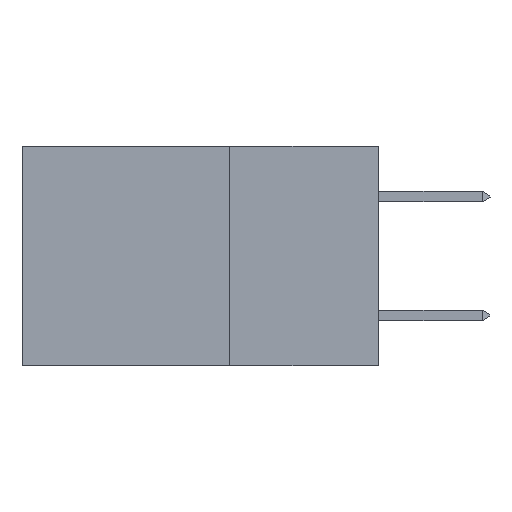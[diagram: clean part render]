
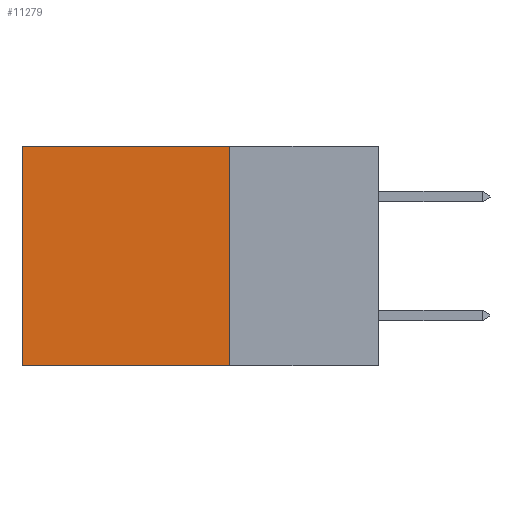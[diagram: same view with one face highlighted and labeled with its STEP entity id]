
A CAD part, left-side view. The second image highlights one B-rep face of the part: STEP entity #11279.
In plain terms, the highlighted planar face has unit normal (-1, 0, 0).
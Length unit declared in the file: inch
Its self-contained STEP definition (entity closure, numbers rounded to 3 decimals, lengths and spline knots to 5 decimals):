
#755 = VERTEX_POINT ( 'NONE', #5905 ) ;
#1146 = DIRECTION ( 'NONE',  ( 0., 0., -1. ) ) ;
#1419 = AXIS2_PLACEMENT_3D ( 'NONE', #7043, #1528, #3377 ) ;
#1528 = DIRECTION ( 'NONE',  ( 1., 0., 0. ) ) ;
#1581 = VECTOR ( 'NONE', #1146, 39.37008 ) ;
#1750 = VECTOR ( 'NONE', #7719, 39.37008 ) ;
#2320 = VECTOR ( 'NONE', #4687, 39.37008 ) ;
#2841 = FACE_OUTER_BOUND ( 'NONE', #6956, .T. ) ;
#2932 = VERTEX_POINT ( 'NONE', #9448 ) ;
#3377 = DIRECTION ( 'NONE',  ( 0., 0., -1. ) ) ;
#3832 = ORIENTED_EDGE ( 'NONE', *, *, #9531, .T. ) ;
#4019 = VERTEX_POINT ( 'NONE', #7221 ) ;
#4687 = DIRECTION ( 'NONE',  ( 0., 1., 0. ) ) ;
#5283 = ORIENTED_EDGE ( 'NONE', *, *, #6499, .F. ) ;
#5541 = ORIENTED_EDGE ( 'NONE', *, *, #7902, .T. ) ;
#5762 = CARTESIAN_POINT ( 'NONE',  ( 0.298, 0.6, 0. ) ) ;
#5766 = CARTESIAN_POINT ( 'NONE',  ( 0.298, 0.25, -0.37 ) ) ;
#5805 = CARTESIAN_POINT ( 'NONE',  ( 0.298, 0.6, -0.37 ) ) ;
#5905 = CARTESIAN_POINT ( 'NONE',  ( 0.298, 0.6, 0. ) ) ;
#6098 = CARTESIAN_POINT ( 'NONE',  ( 0.298, 0.25, 0. ) ) ;
#6193 = PLANE ( 'NONE',  #1419 ) ;
#6499 = EDGE_CURVE ( 'NONE', #2932, #9592, #7952, .T. ) ;
#6956 = EDGE_LOOP ( 'NONE', ( #3832, #5283, #9383, #5541 ) ) ;
#7043 = CARTESIAN_POINT ( 'NONE',  ( 0.298, 0.25, 0. ) ) ;
#7221 = CARTESIAN_POINT ( 'NONE',  ( 0.298, 0.25, 0. ) ) ;
#7719 = DIRECTION ( 'NONE',  ( 0., 1., 0. ) ) ;
#7902 = EDGE_CURVE ( 'NONE', #4019, #755, #9662, .T. ) ;
#7952 = LINE ( 'NONE', #5766, #1750 ) ;
#8038 = CARTESIAN_POINT ( 'NONE',  ( 0.298, 0.25, 0. ) ) ;
#8159 = VECTOR ( 'NONE', #10855, 39.37008 ) ;
#9383 = ORIENTED_EDGE ( 'NONE', *, *, #10842, .F. ) ;
#9448 = CARTESIAN_POINT ( 'NONE',  ( 0.298, 0.25, -0.37 ) ) ;
#9531 = EDGE_CURVE ( 'NONE', #755, #9592, #11811, .T. ) ;
#9592 = VERTEX_POINT ( 'NONE', #5805 ) ;
#9631 = LINE ( 'NONE', #8038, #8159 ) ;
#9662 = LINE ( 'NONE', #6098, #2320 ) ;
#10842 = EDGE_CURVE ( 'NONE', #4019, #2932, #9631, .T. ) ;
#10855 = DIRECTION ( 'NONE',  ( 0., 0., -1. ) ) ;
#11279 = ADVANCED_FACE ( 'NONE', ( #2841 ), #6193, .F. ) ;
#11811 = LINE ( 'NONE', #5762, #1581 ) ;
